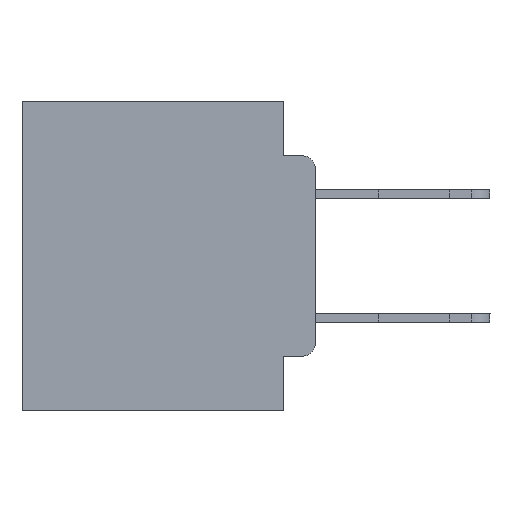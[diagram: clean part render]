
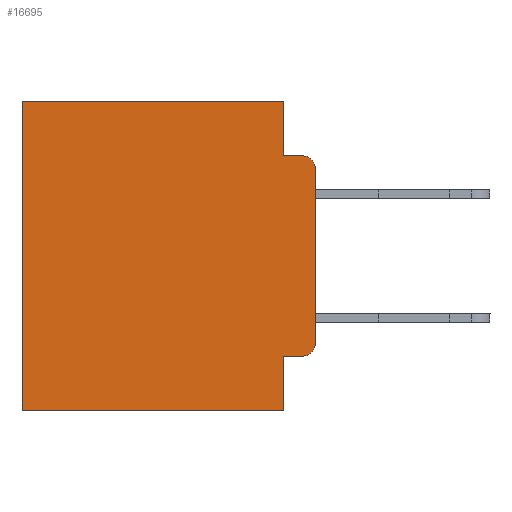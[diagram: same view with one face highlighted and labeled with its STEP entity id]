
A CAD part, left-side view. The second image highlights one B-rep face of the part: STEP entity #16695.
In plain terms, the highlighted planar face has unit normal (-1, 0, 0).
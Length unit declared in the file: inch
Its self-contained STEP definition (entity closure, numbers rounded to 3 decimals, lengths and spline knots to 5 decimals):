
#51 = ORIENTED_EDGE ( 'NONE', *, *, #305, .F. ) ;
#71 = VERTEX_POINT ( 'NONE', #22426 ) ;
#305 = EDGE_CURVE ( 'NONE', #29024, #71, #22422, .T. ) ;
#338 = ORIENTED_EDGE ( 'NONE', *, *, #29074, .T. ) ;
#553 = ORIENTED_EDGE ( 'NONE', *, *, #2627, .F. ) ;
#608 = VERTEX_POINT ( 'NONE', #6795 ) ;
#1060 = VERTEX_POINT ( 'NONE', #5442 ) ;
#1062 = DIRECTION ( 'NONE',  ( 0., 0., -1. ) ) ;
#1199 = ORIENTED_EDGE ( 'NONE', *, *, #26096, .T. ) ;
#1411 = ORIENTED_EDGE ( 'NONE', *, *, #14001, .T. ) ;
#1578 = AXIS2_PLACEMENT_3D ( 'NONE', #21461, #7517, #1062 ) ;
#2627 = EDGE_CURVE ( 'NONE', #1060, #16921, #5616, .T. ) ;
#3210 = CARTESIAN_POINT ( 'NONE',  ( 0.298, 0.051, -0.0885 ) ) ;
#3419 = DIRECTION ( 'NONE',  ( 0., 0., -1. ) ) ;
#3434 = CARTESIAN_POINT ( 'NONE',  ( 0.298, 0., -0.5 ) ) ;
#4645 = DIRECTION ( 'NONE',  ( 0., 0., -1. ) ) ;
#5174 = DIRECTION ( 'NONE',  ( -1., 0., 0. ) ) ;
#5442 = CARTESIAN_POINT ( 'NONE',  ( 0.298, 0.051, -0.0885 ) ) ;
#5616 = LINE ( 'NONE', #3210, #25889 ) ;
#5720 = DIRECTION ( 'NONE',  ( 0., 0., -1. ) ) ;
#5910 = PLANE ( 'NONE',  #26861 ) ;
#6710 = CARTESIAN_POINT ( 'NONE',  ( 0.298, 0.473, 0. ) ) ;
#6795 = CARTESIAN_POINT ( 'NONE',  ( 0.298, 0.473, -0.5 ) ) ;
#7433 = DIRECTION ( 'NONE',  ( 0., 0., -1. ) ) ;
#7463 = CARTESIAN_POINT ( 'NONE',  ( 0.298, 0., -0.3915 ) ) ;
#7517 = DIRECTION ( 'NONE',  ( -1., 0., 0. ) ) ;
#7991 = CARTESIAN_POINT ( 'NONE',  ( 0.298, 0.051, 0. ) ) ;
#8092 = VECTOR ( 'NONE', #19081, 39.37008 ) ;
#9256 = VECTOR ( 'NONE', #10002, 39.37008 ) ;
#9381 = ORIENTED_EDGE ( 'NONE', *, *, #20981, .F. ) ;
#10002 = DIRECTION ( 'NONE',  ( 0., 1., 0. ) ) ;
#10025 = VERTEX_POINT ( 'NONE', #25800 ) ;
#10592 = DIRECTION ( 'NONE',  ( 1., 0., 0. ) ) ;
#10695 = LINE ( 'NONE', #7991, #13693 ) ;
#11335 = EDGE_CURVE ( 'NONE', #23200, #1060, #10695, .T. ) ;
#11740 = VERTEX_POINT ( 'NONE', #27773 ) ;
#12961 = FACE_OUTER_BOUND ( 'NONE', #18318, .T. ) ;
#13072 = VECTOR ( 'NONE', #5720, 39.37008 ) ;
#13113 = LINE ( 'NONE', #17910, #20925 ) ;
#13693 = VECTOR ( 'NONE', #3419, 39.37008 ) ;
#14001 = EDGE_CURVE ( 'NONE', #11740, #608, #20413, .T. ) ;
#14314 = CARTESIAN_POINT ( 'NONE',  ( 0.298, 0.051, -0.4115 ) ) ;
#14428 = CARTESIAN_POINT ( 'NONE',  ( 0.298, 0.02, -0.1085 ) ) ;
#14962 = VECTOR ( 'NONE', #23600, 39.37008 ) ;
#14970 = EDGE_CURVE ( 'NONE', #10025, #15376, #26874, .T. ) ;
#15105 = ORIENTED_EDGE ( 'NONE', *, *, #11335, .F. ) ;
#15376 = VERTEX_POINT ( 'NONE', #7463 ) ;
#16352 = ORIENTED_EDGE ( 'NONE', *, *, #29179, .T. ) ;
#16695 = ADVANCED_FACE ( 'NONE', ( #12961 ), #5910, .F. ) ;
#16921 = VERTEX_POINT ( 'NONE', #17838 ) ;
#17838 = CARTESIAN_POINT ( 'NONE',  ( 0.298, 0.02, -0.0885 ) ) ;
#17867 = VERTEX_POINT ( 'NONE', #26495 ) ;
#17910 = CARTESIAN_POINT ( 'NONE',  ( 0.298, 0.051, -0.4115 ) ) ;
#18318 = EDGE_LOOP ( 'NONE', ( #23934, #338, #553, #15105, #16352, #1411, #9381, #51, #18731, #1199 ) ) ;
#18731 = ORIENTED_EDGE ( 'NONE', *, *, #23785, .T. ) ;
#18782 = CIRCLE ( 'NONE', #27474, 0.02 ) ;
#19081 = DIRECTION ( 'NONE',  ( 0., 1., 0. ) ) ;
#19393 = CARTESIAN_POINT ( 'NONE',  ( 0.298, 0., 0. ) ) ;
#19755 = CARTESIAN_POINT ( 'NONE',  ( 0.298, 0., 0. ) ) ;
#20413 = LINE ( 'NONE', #6710, #26792 ) ;
#20925 = VECTOR ( 'NONE', #24748, 39.37008 ) ;
#20981 = EDGE_CURVE ( 'NONE', #71, #608, #23500, .T. ) ;
#21329 = CARTESIAN_POINT ( 'NONE',  ( 0.298, 0.051, 0. ) ) ;
#21461 = CARTESIAN_POINT ( 'NONE',  ( 0.298, 0.02, -0.3915 ) ) ;
#22422 = LINE ( 'NONE', #21329, #14962 ) ;
#22426 = CARTESIAN_POINT ( 'NONE',  ( 0.298, 0.051, -0.5 ) ) ;
#23200 = VERTEX_POINT ( 'NONE', #24867 ) ;
#23500 = LINE ( 'NONE', #3434, #9256 ) ;
#23600 = DIRECTION ( 'NONE',  ( 0., 0., -1. ) ) ;
#23785 = EDGE_CURVE ( 'NONE', #29024, #17867, #13113, .T. ) ;
#23792 = DIRECTION ( 'NONE',  ( 0., -1., 0. ) ) ;
#23934 = ORIENTED_EDGE ( 'NONE', *, *, #14970, .F. ) ;
#23966 = CIRCLE ( 'NONE', #1578, 0.02 ) ;
#24748 = DIRECTION ( 'NONE',  ( 0., -1., 0. ) ) ;
#24867 = CARTESIAN_POINT ( 'NONE',  ( 0.298, 0.051, 0. ) ) ;
#25800 = CARTESIAN_POINT ( 'NONE',  ( 0.298, 0., -0.1085 ) ) ;
#25889 = VECTOR ( 'NONE', #23792, 39.37008 ) ;
#26096 = EDGE_CURVE ( 'NONE', #17867, #15376, #23966, .T. ) ;
#26495 = CARTESIAN_POINT ( 'NONE',  ( 0.298, 0.02, -0.4115 ) ) ;
#26550 = CARTESIAN_POINT ( 'NONE',  ( 0.298, 0., 0. ) ) ;
#26641 = DIRECTION ( 'NONE',  ( 0., 0., -1. ) ) ;
#26792 = VECTOR ( 'NONE', #4645, 39.37008 ) ;
#26861 = AXIS2_PLACEMENT_3D ( 'NONE', #26550, #10592, #26641 ) ;
#26874 = LINE ( 'NONE', #19755, #13072 ) ;
#27250 = LINE ( 'NONE', #19393, #8092 ) ;
#27474 = AXIS2_PLACEMENT_3D ( 'NONE', #14428, #5174, #7433 ) ;
#27773 = CARTESIAN_POINT ( 'NONE',  ( 0.298, 0.473, 0. ) ) ;
#29024 = VERTEX_POINT ( 'NONE', #14314 ) ;
#29074 = EDGE_CURVE ( 'NONE', #10025, #16921, #18782, .T. ) ;
#29179 = EDGE_CURVE ( 'NONE', #23200, #11740, #27250, .T. ) ;
